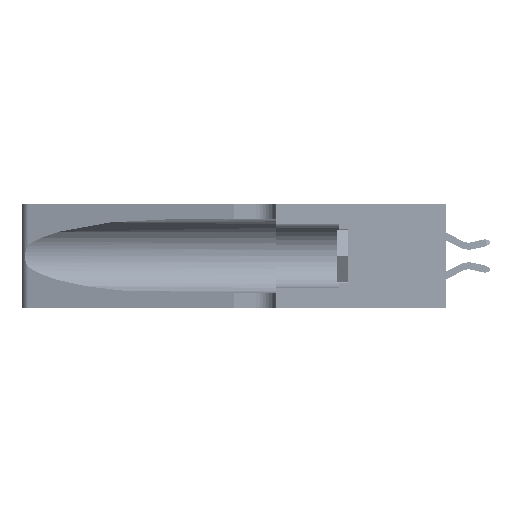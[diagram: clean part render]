
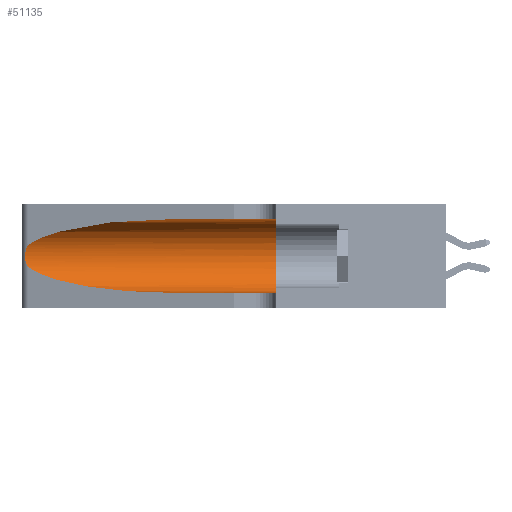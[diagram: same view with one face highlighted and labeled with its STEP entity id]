
A CAD part, left-side view. The second image highlights one B-rep face of the part: STEP entity #51135.
In plain terms, the highlighted cylindrical face has radius 3.308 mm (diameter 6.617 mm), a partial arc.
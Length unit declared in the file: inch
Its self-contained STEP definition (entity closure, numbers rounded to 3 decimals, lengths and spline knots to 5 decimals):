
#1756 = AXIS2_PLACEMENT_3D ( 'NONE', #35397, #22806, #15153 ) ;
#6060 = CARTESIAN_POINT ( 'NONE',  ( 0.1305, 0.35, 0.05475 ) ) ;
#8046 = CARTESIAN_POINT ( 'NONE',  ( 0.2373, 1.15595, 0.08982 ) ) ;
#8118 = CARTESIAN_POINT ( 'NONE',  ( 0.25487, 1.22718, 0.14631 ) ) ;
#8304 = LINE ( 'NONE', #30979, #11418 ) ;
#8638 = CARTESIAN_POINT ( 'NONE',  ( 0.25789, 1.23486, 0.15765 ) ) ;
#9601 = CARTESIAN_POINT ( 'NONE',  ( 0.1305, 1.61858, 0.31525 ) ) ;
#10029 = EDGE_CURVE ( 'NONE', #37107, #16396, #43545, .T. ) ;
#11418 = VECTOR ( 'NONE', #31154, 39.37008 ) ;
#11939 = CYLINDRICAL_SURFACE ( 'NONE', #28758, 0.13025 ) ;
#12561 = CARTESIAN_POINT ( 'NONE',  ( 0.1305, 0.72297, 0.31525 ) ) ;
#12666 = CARTESIAN_POINT ( 'NONE',  ( 0.25787, 1.23484, 0.2124 ) ) ;
#13369 = VERTEX_POINT ( 'NONE', #22306 ) ;
#14350 = CARTESIAN_POINT ( 'NONE',  ( 0.1305, 0.72297, 0.05475 ) ) ;
#14409 = EDGE_CURVE ( 'NONE', #13369, #36158, #14832, .T. ) ;
#14832 = B_SPLINE_CURVE_WITH_KNOTS ( 'NONE', 3,
 ( #24319, #23976, #44409, #12666, #32554, #24155, #28525, #44583, #16670, #16487, #8638, #15965, #39878, #8118 ),
 .UNSPECIFIED., .F., .F.,
 ( 4, 2, 2, 2, 2, 2, 4 ),
 ( 0., 0.00027, 0.00053, 0.00107, 0.0016, 0.00187, 0.00214 ),
 .UNSPECIFIED. ) ;
#15045 = CARTESIAN_POINT ( 'NONE',  ( 0.1305, 0.35, 0.31525 ) ) ;
#15153 = DIRECTION ( 'NONE',  ( 0., 0., 1. ) ) ;
#15742 = VERTEX_POINT ( 'NONE', #12561 ) ;
#15965 = CARTESIAN_POINT ( 'NONE',  ( 0.25639, 1.23186, 0.15144 ) ) ;
#16240 = CARTESIAN_POINT ( 'NONE',  ( 0.25487, 1.22718, 0.14631 ) ) ;
#16396 = VERTEX_POINT ( 'NONE', #6060 ) ;
#16487 = CARTESIAN_POINT ( 'NONE',  ( 0.25856, 1.23593, 0.16098 ) ) ;
#16670 = CARTESIAN_POINT ( 'NONE',  ( 0.26017, 1.23833, 0.17102 ) ) ;
#17289 = CARTESIAN_POINT ( 'NONE',  ( 0.1305, 0.72297, 0.05475 ) ) ;
#17637 = DIRECTION ( 'NONE',  ( 0., -1., 0. ) ) ;
#19183 = CARTESIAN_POINT ( 'NONE',  ( 0.25487, 1.22718, 0.22369 ) ) ;
#20228 = DIRECTION ( 'NONE',  ( 0., 0., -1. ) ) ;
#22306 = CARTESIAN_POINT ( 'NONE',  ( 0.25487, 1.22718, 0.22369 ) ) ;
#22517 = FACE_OUTER_BOUND ( 'NONE', #45311, .T. ) ;
#22806 = DIRECTION ( 'NONE',  ( 0., 1., 0. ) ) ;
#23976 = CARTESIAN_POINT ( 'NONE',  ( 0.25555, 1.22994, 0.2215 ) ) ;
#24155 = CARTESIAN_POINT ( 'NONE',  ( 0.26018, 1.23835, 0.19895 ) ) ;
#24319 = CARTESIAN_POINT ( 'NONE',  ( 0.25487, 1.22718, 0.22369 ) ) ;
#26809 = ORIENTED_EDGE ( 'NONE', *, *, #34872, .T. ) ;
#27737 = VERTEX_POINT ( 'NONE', #14350 ) ;
#28248 = CARTESIAN_POINT ( 'NONE',  ( 0.1305, 1.61858, 0.185 ) ) ;
#28525 = CARTESIAN_POINT ( 'NONE',  ( 0.26075, 1.23896, 0.19203 ) ) ;
#28758 = AXIS2_PLACEMENT_3D ( 'NONE', #28248, #44150, #20228 ) ;
#30979 = CARTESIAN_POINT ( 'NONE',  ( 0.1305, 1.61858, 0.05475 ) ) ;
#31154 = DIRECTION ( 'NONE',  ( 0., -1., 0. ) ) ;
#32448 = CARTESIAN_POINT ( 'NONE',  ( 0.25487, 1.22718, 0.14631 ) ) ;
#32554 = CARTESIAN_POINT ( 'NONE',  ( 0.25854, 1.2359, 0.20912 ) ) ;
#32744 =( BOUNDED_CURVE ( )  B_SPLINE_CURVE ( 3, ( #16240, #8046, #40669, #17289 ),
 .UNSPECIFIED., .F., .F. ) 
 B_SPLINE_CURVE_WITH_KNOTS ( ( 4, 4 ),
 ( 3.44316, 4.71239 ),
 .UNSPECIFIED. ) 
 CURVE ( )  GEOMETRIC_REPRESENTATION_ITEM ( )  RATIONAL_B_SPLINE_CURVE ( ( 1., 0.87, 0.87, 1. ) ) 
 REPRESENTATION_ITEM ( '' )  );
#33805 = ORIENTED_EDGE ( 'NONE', *, *, #10029, .F. ) ;
#34563 = CARTESIAN_POINT ( 'NONE',  ( 0.18966, 0.96281, 0.31525 ) ) ;
#34826 = ORIENTED_EDGE ( 'NONE', *, *, #37618, .F. ) ;
#34872 = EDGE_CURVE ( 'NONE', #27737, #16396, #8304, .T. ) ;
#34906 = CARTESIAN_POINT ( 'NONE',  ( 0.1305, 0.72297, 0.31525 ) ) ;
#35397 = CARTESIAN_POINT ( 'NONE',  ( 0.1305, 0.35, 0.185 ) ) ;
#36158 = VERTEX_POINT ( 'NONE', #32448 ) ;
#37107 = VERTEX_POINT ( 'NONE', #15045 ) ;
#37618 = EDGE_CURVE ( 'NONE', #15742, #37107, #41077, .T. ) ;
#39062 = CARTESIAN_POINT ( 'NONE',  ( 0.2373, 1.15595, 0.28018 ) ) ;
#39878 = CARTESIAN_POINT ( 'NONE',  ( 0.25555, 1.22993, 0.14849 ) ) ;
#40669 = CARTESIAN_POINT ( 'NONE',  ( 0.18966, 0.96281, 0.05475 ) ) ;
#41077 = LINE ( 'NONE', #9601, #51065 ) ;
#43545 = CIRCLE ( 'NONE', #1756, 0.13025 ) ;
#43592 =( BOUNDED_CURVE ( )  B_SPLINE_CURVE ( 3, ( #34906, #34563, #39062, #19183 ),
 .UNSPECIFIED., .F., .F. ) 
 B_SPLINE_CURVE_WITH_KNOTS ( ( 4, 4 ),
 ( 1.5708, 2.84003 ),
 .UNSPECIFIED. ) 
 CURVE ( )  GEOMETRIC_REPRESENTATION_ITEM ( )  RATIONAL_B_SPLINE_CURVE ( ( 1., 0.87, 0.87, 1. ) ) 
 REPRESENTATION_ITEM ( '' )  );
#44150 = DIRECTION ( 'NONE',  ( 0., -1., 0. ) ) ;
#44186 = ORIENTED_EDGE ( 'NONE', *, *, #14409, .T. ) ;
#44409 = CARTESIAN_POINT ( 'NONE',  ( 0.25639, 1.23184, 0.21858 ) ) ;
#44583 = CARTESIAN_POINT ( 'NONE',  ( 0.26075, 1.23896, 0.178 ) ) ;
#45256 = ORIENTED_EDGE ( 'NONE', *, *, #45895, .T. ) ;
#45311 = EDGE_LOOP ( 'NONE', ( #45256, #44186, #50894, #26809, #33805, #34826 ) ) ;
#45895 = EDGE_CURVE ( 'NONE', #15742, #13369, #43592, .T. ) ;
#47468 = EDGE_CURVE ( 'NONE', #36158, #27737, #32744, .T. ) ;
#50894 = ORIENTED_EDGE ( 'NONE', *, *, #47468, .T. ) ;
#51065 = VECTOR ( 'NONE', #17637, 39.37008 ) ;
#51135 = ADVANCED_FACE ( 'NONE', ( #22517 ), #11939, .F. ) ;
